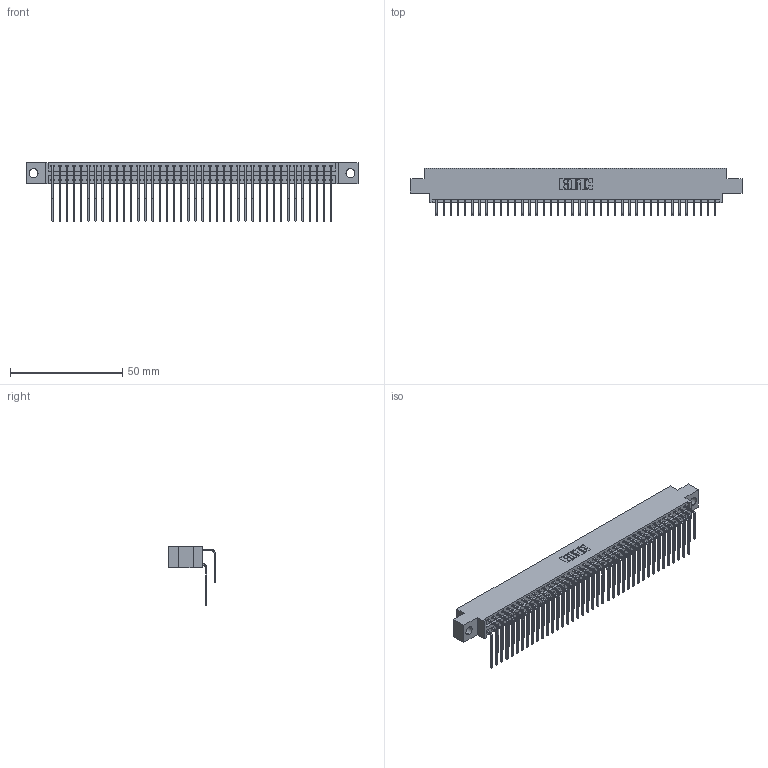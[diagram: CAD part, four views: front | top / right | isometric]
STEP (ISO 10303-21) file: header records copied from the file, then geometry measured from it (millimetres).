
FILE_DESCRIPTION (( 'STEP AP203' ), '1' );
FILE_NAME ('396-080-559-804.STEP', '2018-09-09T21:50:10', ( '' ), ( '' ), 'SwSTEP 2.0', 'SolidWorks 2016', '' );
FILE_SCHEMA (( 'CONFIG_CONTROL_DESIGN' ));
Length unit declared in the file: inch
Products named in the file (4): 396-080-559-804; 346 Part_0.170 Offset - 0.156 Dia-TH; 345-292-001_558 559 Tail - 1; 345-292-001_559 Tail - 2
Assembly tree (81 placements, depth 2):
  396-080-559-804
    346 Part_0.170 Offset - 0.156 Dia-TH
    345-292-001_558 559 Tail - 1  x40
    345-292-001_559 Tail - 2  x40
Bounding box: 147.57 x 20.89 x 26.16 mm (x, y, z)
Volume: 14593.8 mm3; surface area: 22235.7 mm2
Topology: 81 solids, 81 shells, 4446 faces, 13221 edges, 8706 vertices
Faces by surface type: plane 3040, cylinder 1406
Entity records: 28293 total; most frequent: CARTESIAN_POINT 4719, ORIENTED_EDGE 4602, DIRECTION 4181, EDGE_CURVE 2301, VECTOR 1969, LINE 1969, VERTEX_POINT 1530, AXIS2_PLACEMENT_3D 1106
